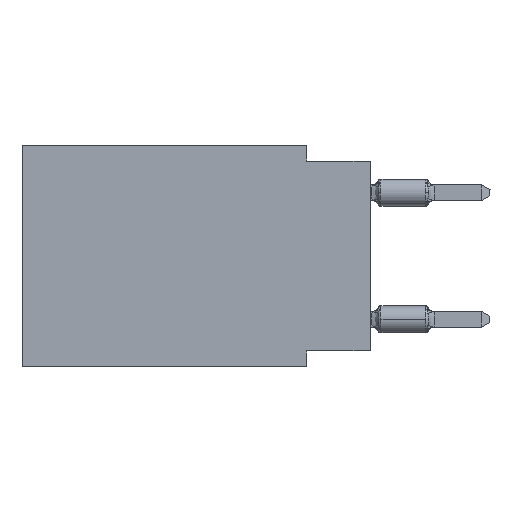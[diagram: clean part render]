
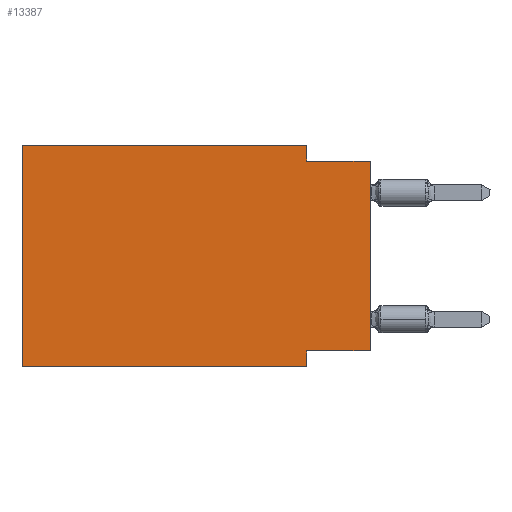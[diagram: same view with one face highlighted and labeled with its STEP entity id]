
A CAD part, left-side view. The second image highlights one B-rep face of the part: STEP entity #13387.
In plain terms, the highlighted planar face has unit normal (-1, 0, 0).
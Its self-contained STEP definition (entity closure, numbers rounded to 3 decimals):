
#94 = DIRECTION ( 'NONE',  ( 0., -1., 0. ) ) ;
#313 = VERTEX_POINT ( 'NONE', #5219 ) ;
#337 = ORIENTED_EDGE ( 'NONE', *, *, #9378, .F. ) ;
#847 = CARTESIAN_POINT ( 'NONE',  ( 0., 2.54, -8.89 ) ) ;
#1269 = CARTESIAN_POINT ( 'NONE',  ( 0., 13.97, 0. ) ) ;
#1874 = VERTEX_POINT ( 'NONE', #1269 ) ;
#2587 = AXIS2_PLACEMENT_3D ( 'NONE', #24754, #4193, #17553 ) ;
#3079 = EDGE_CURVE ( 'NONE', #9450, #6685, #18647, .T. ) ;
#4193 = DIRECTION ( 'NONE',  ( 1., 0., 0. ) ) ;
#4194 = EDGE_CURVE ( 'NONE', #6685, #313, #6665, .T. ) ;
#4204 = ORIENTED_EDGE ( 'NONE', *, *, #5528, .F. ) ;
#4470 = CARTESIAN_POINT ( 'NONE',  ( 0., 2.54, 0. ) ) ;
#4752 = CARTESIAN_POINT ( 'NONE',  ( 0., 13.97, 0. ) ) ;
#4807 = DIRECTION ( 'NONE',  ( 0., 0., 1. ) ) ;
#5219 = CARTESIAN_POINT ( 'NONE',  ( 0., 0., -0.635 ) ) ;
#5528 = EDGE_CURVE ( 'NONE', #19066, #19074, #29118, .T. ) ;
#5814 = ORIENTED_EDGE ( 'NONE', *, *, #18575, .T. ) ;
#6408 = ORIENTED_EDGE ( 'NONE', *, *, #27641, .F. ) ;
#6418 = DIRECTION ( 'NONE',  ( 0., 0., -1. ) ) ;
#6665 = LINE ( 'NONE', #13268, #21449 ) ;
#6685 = VERTEX_POINT ( 'NONE', #9539 ) ;
#7095 = DIRECTION ( 'NONE',  ( 0., 0., -1. ) ) ;
#7694 = VECTOR ( 'NONE', #7801, 1000. ) ;
#7801 = DIRECTION ( 'NONE',  ( 0., 0., 1. ) ) ;
#8094 = CARTESIAN_POINT ( 'NONE',  ( 0., 0., 0. ) ) ;
#8591 = DIRECTION ( 'NONE',  ( 0., -1., 0. ) ) ;
#8718 = CARTESIAN_POINT ( 'NONE',  ( 0., 2.54, -8.255 ) ) ;
#9378 = EDGE_CURVE ( 'NONE', #19074, #9615, #20082, .T. ) ;
#9450 = VERTEX_POINT ( 'NONE', #4470 ) ;
#9539 = CARTESIAN_POINT ( 'NONE',  ( 0., 2.54, -0.635 ) ) ;
#9615 = VERTEX_POINT ( 'NONE', #847 ) ;
#10159 = EDGE_LOOP ( 'NONE', ( #12279, #21138, #13538, #6408, #10834, #5814, #337, #4204 ) ) ;
#10574 = VECTOR ( 'NONE', #8591, 1000. ) ;
#10651 = VECTOR ( 'NONE', #94, 1000. ) ;
#10834 = ORIENTED_EDGE ( 'NONE', *, *, #11055, .F. ) ;
#10922 = CARTESIAN_POINT ( 'NONE',  ( 0., 2.54, -8.89 ) ) ;
#10964 = CARTESIAN_POINT ( 'NONE',  ( 0., 0., -8.255 ) ) ;
#11055 = EDGE_CURVE ( 'NONE', #22389, #1874, #18925, .T. ) ;
#11269 = EDGE_CURVE ( 'NONE', #19066, #313, #28678, .T. ) ;
#12279 = ORIENTED_EDGE ( 'NONE', *, *, #11269, .T. ) ;
#13268 = CARTESIAN_POINT ( 'NONE',  ( 0., 0., -0.635 ) ) ;
#13387 = ADVANCED_FACE ( 'NONE', ( #15601 ), #22794, .F. ) ;
#13538 = ORIENTED_EDGE ( 'NONE', *, *, #3079, .F. ) ;
#13712 = DIRECTION ( 'NONE',  ( 0., -1., 0. ) ) ;
#15601 = FACE_OUTER_BOUND ( 'NONE', #10159, .T. ) ;
#15889 = DIRECTION ( 'NONE',  ( 0., 1., 0. ) ) ;
#17553 = DIRECTION ( 'NONE',  ( 0., 0., -1. ) ) ;
#18575 = EDGE_CURVE ( 'NONE', #22389, #9615, #20007, .T. ) ;
#18647 = LINE ( 'NONE', #20757, #26194 ) ;
#18925 = LINE ( 'NONE', #20730, #21586 ) ;
#19066 = VERTEX_POINT ( 'NONE', #10964 ) ;
#19074 = VERTEX_POINT ( 'NONE', #8718 ) ;
#19672 = CARTESIAN_POINT ( 'NONE',  ( 0., 13.97, -8.89 ) ) ;
#20007 = LINE ( 'NONE', #24208, #10574 ) ;
#20082 = LINE ( 'NONE', #10922, #28921 ) ;
#20400 = CARTESIAN_POINT ( 'NONE',  ( 0., 0., -8.255 ) ) ;
#20679 = LINE ( 'NONE', #4752, #10651 ) ;
#20730 = CARTESIAN_POINT ( 'NONE',  ( 0., 13.97, 0. ) ) ;
#20757 = CARTESIAN_POINT ( 'NONE',  ( 0., 2.54, 0. ) ) ;
#21138 = ORIENTED_EDGE ( 'NONE', *, *, #4194, .F. ) ;
#21449 = VECTOR ( 'NONE', #13712, 1000. ) ;
#21586 = VECTOR ( 'NONE', #4807, 1000. ) ;
#22389 = VERTEX_POINT ( 'NONE', #19672 ) ;
#22794 = PLANE ( 'NONE',  #2587 ) ;
#24208 = CARTESIAN_POINT ( 'NONE',  ( 0., 13.97, -8.89 ) ) ;
#24754 = CARTESIAN_POINT ( 'NONE',  ( 0., 13.97, 0. ) ) ;
#26194 = VECTOR ( 'NONE', #7095, 1000. ) ;
#27641 = EDGE_CURVE ( 'NONE', #1874, #9450, #20679, .T. ) ;
#27866 = VECTOR ( 'NONE', #15889, 1000. ) ;
#28678 = LINE ( 'NONE', #8094, #7694 ) ;
#28921 = VECTOR ( 'NONE', #6418, 1000. ) ;
#29118 = LINE ( 'NONE', #20400, #27866 ) ;
